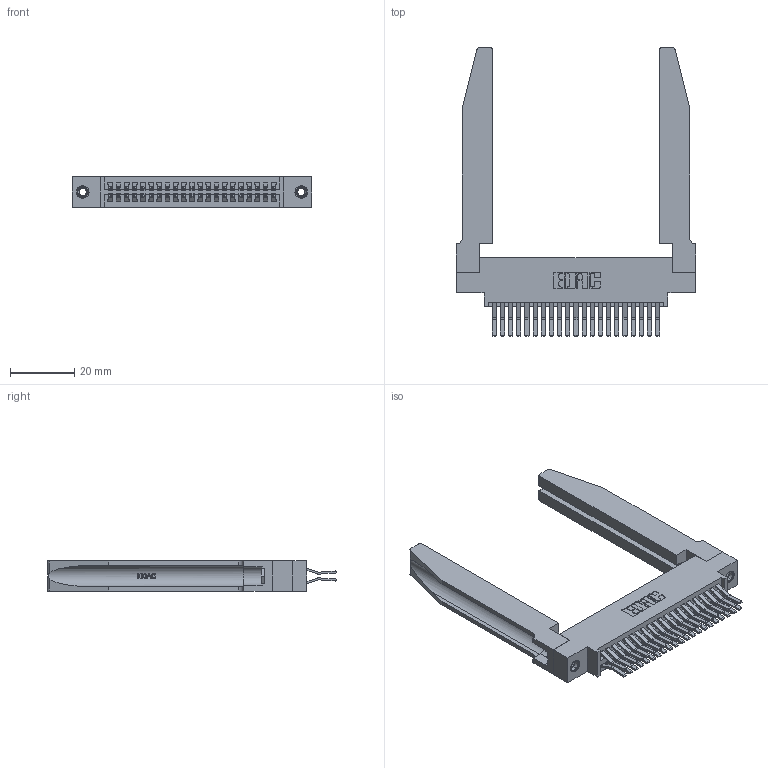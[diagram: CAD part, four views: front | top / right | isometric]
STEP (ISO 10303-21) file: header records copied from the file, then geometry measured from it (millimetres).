
FILE_DESCRIPTION (( 'STEP AP203' ), '1' );
FILE_NAME ('345-042-560-878.STEP', '2019-10-28T22:47:44', ( '' ), ( '' ), 'SwSTEP 2.0', 'SolidWorks 2016', '' );
FILE_SCHEMA (( 'CONFIG_CONTROL_DESIGN' ));
Length unit declared in the file: inch
Products named in the file (5): 345 Part_0.170 Offset - 0.156 Dia-TH; 345-292-001_560 Tail; 345-220-078_345-220-078; 345-042-560-878; 345-250-001_345-250-001-102
Assembly tree (47 placements, depth 2):
  345-042-560-878
    345 Part_0.170 Offset - 0.156 Dia-TH
    345-292-001_560 Tail  x42
    345-250-001_345-250-001-102  x2
    345-220-078_345-220-078  x2
Bounding box: 74.57 x 89.72 x 9.4 mm (x, y, z)
Volume: 14981.6 mm3; surface area: 17942.6 mm2
Topology: 47 solids, 47 shells, 2548 faces, 7471 edges, 4914 vertices
Faces by surface type: plane 1612, cylinder 884, bspline 36, cone 12, torus 4
Entity records: 24264 total; most frequent: CARTESIAN_POINT 5007, ORIENTED_EDGE 3838, DIRECTION 3437, EDGE_CURVE 1919, LINE 1605, VECTOR 1605, VERTEX_POINT 1272, AXIS2_PLACEMENT_3D 916
